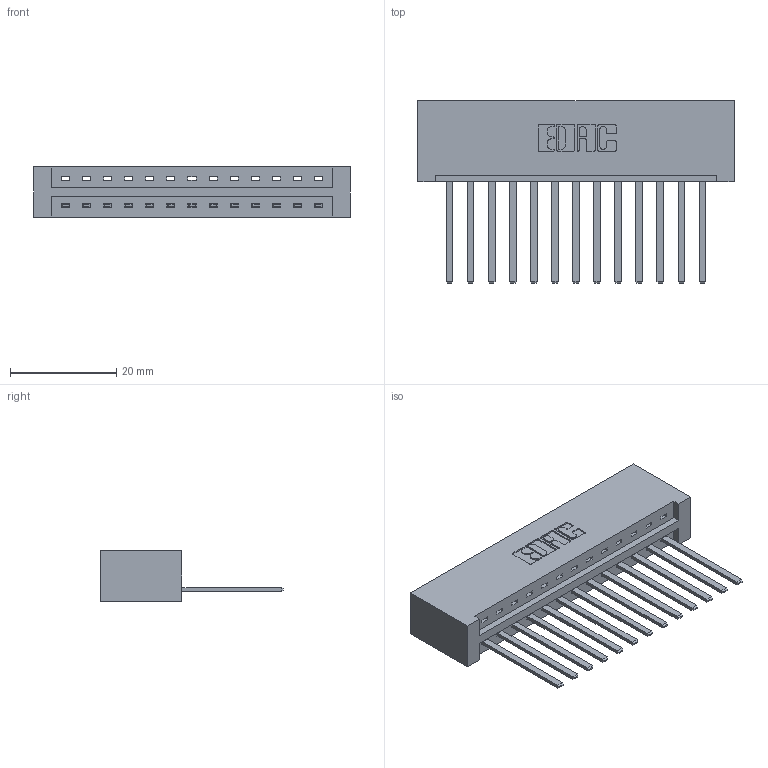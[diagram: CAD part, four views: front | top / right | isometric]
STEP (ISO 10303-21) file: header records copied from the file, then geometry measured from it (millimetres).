
FILE_DESCRIPTION (( 'STEP AP203' ), '1' );
FILE_NAME ('387-013-544-101.STEP', '2018-09-11T00:42:34', ( '' ), ( '' ), 'SwSTEP 2.0', 'SolidWorks 2016', '' );
FILE_SCHEMA (( 'CONFIG_CONTROL_DESIGN' ));
Length unit declared in the file: inch
Products named in the file (3): 337 Part_No Mounting Lugs; 345-292-001_345-293-144; 387-013-544-101
Assembly tree (14 placements, depth 2):
  387-013-544-101
    337 Part_No Mounting Lugs
    345-292-001_345-293-144  x13
Bounding box: 59.39 x 34.3 x 9.4 mm (x, y, z)
Volume: 6698.5 mm3; surface area: 7237.6 mm2
Topology: 14 solids, 14 shells, 834 faces, 2497 edges, 1646 vertices
Faces by surface type: plane 612, cylinder 222
Entity records: 12953 total; most frequent: CARTESIAN_POINT 2261, ORIENTED_EDGE 2210, DIRECTION 1951, EDGE_CURVE 1105, LINE 989, VECTOR 989, VERTEX_POINT 734, AXIS2_PLACEMENT_3D 481
